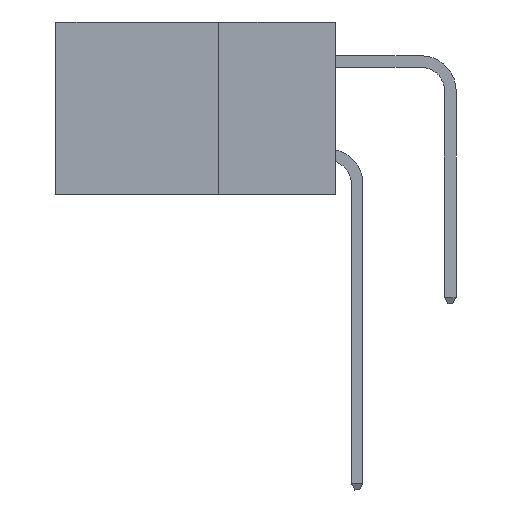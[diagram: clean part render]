
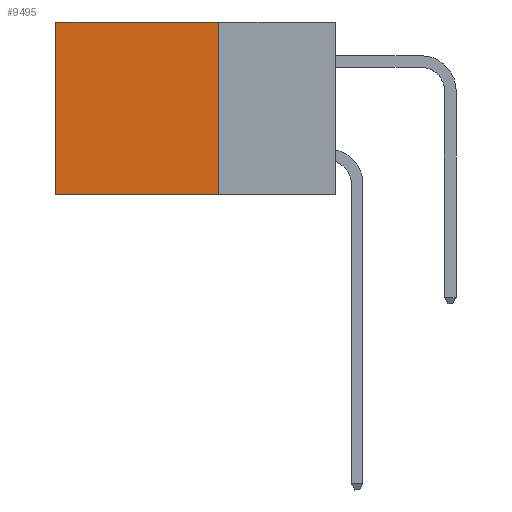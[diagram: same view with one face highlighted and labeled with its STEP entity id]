
A CAD part, left-side view. The second image highlights one B-rep face of the part: STEP entity #9495.
In plain terms, the highlighted planar face has unit normal (-1, 0, 0).
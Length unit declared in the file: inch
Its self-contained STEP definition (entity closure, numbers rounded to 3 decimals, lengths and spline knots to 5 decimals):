
#244 = CARTESIAN_POINT ( 'NONE',  ( 0.2875, 0.25, -0.37 ) ) ;
#405 = DIRECTION ( 'NONE',  ( 0., 0., -1. ) ) ;
#3039 = EDGE_CURVE ( 'NONE', #32021, #30122, #34938, .T. ) ;
#4083 = CARTESIAN_POINT ( 'NONE',  ( 0.2875, 0.25, 0. ) ) ;
#4324 = VECTOR ( 'NONE', #405, 39.37008 ) ;
#5626 = VECTOR ( 'NONE', #19739, 39.37008 ) ;
#5955 = CARTESIAN_POINT ( 'NONE',  ( 0.2875, 0.25, 0. ) ) ;
#6174 = VERTEX_POINT ( 'NONE', #5955 ) ;
#8076 = DIRECTION ( 'NONE',  ( 0., 1., 0. ) ) ;
#8085 = CARTESIAN_POINT ( 'NONE',  ( 0.2875, 0.6, -0.37 ) ) ;
#9495 = ADVANCED_FACE ( 'NONE', ( #34547 ), #27368, .F. ) ;
#11752 = EDGE_CURVE ( 'NONE', #37212, #30122, #22084, .T. ) ;
#13378 = ORIENTED_EDGE ( 'NONE', *, *, #35872, .T. ) ;
#14885 = DIRECTION ( 'NONE',  ( 0., 0., -1. ) ) ;
#15137 = VECTOR ( 'NONE', #8076, 39.37008 ) ;
#16970 = LINE ( 'NONE', #28644, #15137 ) ;
#18802 = DIRECTION ( 'NONE',  ( 0., 0., -1. ) ) ;
#19739 = DIRECTION ( 'NONE',  ( 0., 1., 0. ) ) ;
#20116 = CARTESIAN_POINT ( 'NONE',  ( 0.2875, 0.6, 0. ) ) ;
#22084 = LINE ( 'NONE', #244, #5626 ) ;
#24418 = DIRECTION ( 'NONE',  ( 1., 0., 0. ) ) ;
#26680 = CARTESIAN_POINT ( 'NONE',  ( 0.2875, 0.6, 0. ) ) ;
#26951 = EDGE_LOOP ( 'NONE', ( #31336, #35618, #31334, #13378 ) ) ;
#27368 = PLANE ( 'NONE',  #33985 ) ;
#27822 = EDGE_CURVE ( 'NONE', #6174, #37212, #32703, .T. ) ;
#28644 = CARTESIAN_POINT ( 'NONE',  ( 0.2875, 0.25, 0. ) ) ;
#30122 = VERTEX_POINT ( 'NONE', #8085 ) ;
#30197 = CARTESIAN_POINT ( 'NONE',  ( 0.2875, 0.25, 0. ) ) ;
#30902 = VECTOR ( 'NONE', #14885, 39.37008 ) ;
#31334 = ORIENTED_EDGE ( 'NONE', *, *, #27822, .F. ) ;
#31336 = ORIENTED_EDGE ( 'NONE', *, *, #3039, .T. ) ;
#32021 = VERTEX_POINT ( 'NONE', #20116 ) ;
#32703 = LINE ( 'NONE', #4083, #30902 ) ;
#33985 = AXIS2_PLACEMENT_3D ( 'NONE', #30197, #24418, #18802 ) ;
#34547 = FACE_OUTER_BOUND ( 'NONE', #26951, .T. ) ;
#34938 = LINE ( 'NONE', #26680, #4324 ) ;
#35010 = CARTESIAN_POINT ( 'NONE',  ( 0.2875, 0.25, -0.37 ) ) ;
#35618 = ORIENTED_EDGE ( 'NONE', *, *, #11752, .F. ) ;
#35872 = EDGE_CURVE ( 'NONE', #6174, #32021, #16970, .T. ) ;
#37212 = VERTEX_POINT ( 'NONE', #35010 ) ;
